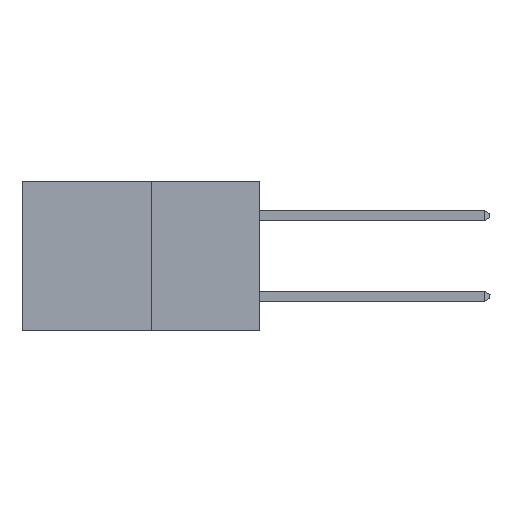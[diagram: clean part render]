
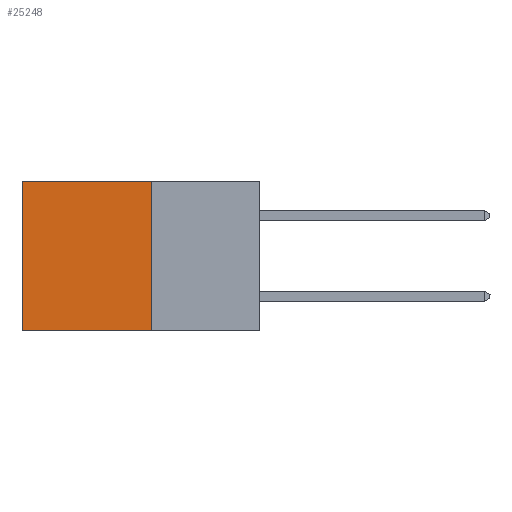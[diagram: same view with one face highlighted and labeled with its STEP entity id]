
A CAD part, left-side view. The second image highlights one B-rep face of the part: STEP entity #25248.
In plain terms, the highlighted planar face has unit normal (-1, 0, 0).
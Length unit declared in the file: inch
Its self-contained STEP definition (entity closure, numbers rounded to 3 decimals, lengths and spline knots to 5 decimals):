
#988 = CARTESIAN_POINT ( 'NONE',  ( 0.277, 0.27, -0.37 ) ) ;
#2246 = VECTOR ( 'NONE', #14841, 39.37008 ) ;
#3165 = AXIS2_PLACEMENT_3D ( 'NONE', #18315, #5723, #20371 ) ;
#3488 = ORIENTED_EDGE ( 'NONE', *, *, #22690, .F. ) ;
#4357 = CARTESIAN_POINT ( 'NONE',  ( 0.277, 0.27, 0. ) ) ;
#5223 = VERTEX_POINT ( 'NONE', #17299 ) ;
#5723 = DIRECTION ( 'NONE',  ( 1., 0., 0. ) ) ;
#6029 = VERTEX_POINT ( 'NONE', #8067 ) ;
#6494 = DIRECTION ( 'NONE',  ( 0., 1., 0. ) ) ;
#6963 = CARTESIAN_POINT ( 'NONE',  ( 0.277, 0.27, -0.37 ) ) ;
#7068 = EDGE_LOOP ( 'NONE', ( #21282, #3488, #13010, #15173 ) ) ;
#7414 = CARTESIAN_POINT ( 'NONE',  ( 0.277, 0.59, -0.37 ) ) ;
#7594 = EDGE_CURVE ( 'NONE', #5223, #8471, #8570, .T. ) ;
#8067 = CARTESIAN_POINT ( 'NONE',  ( 0.277, 0.27, 0. ) ) ;
#8471 = VERTEX_POINT ( 'NONE', #7414 ) ;
#8570 = LINE ( 'NONE', #12725, #2246 ) ;
#9075 = DIRECTION ( 'NONE',  ( 0., 0., -1. ) ) ;
#10999 = VECTOR ( 'NONE', #11600, 39.37008 ) ;
#11600 = DIRECTION ( 'NONE',  ( 0., 1., 0. ) ) ;
#12725 = CARTESIAN_POINT ( 'NONE',  ( 0.277, 0.59, -0.37 ) ) ;
#13010 = ORIENTED_EDGE ( 'NONE', *, *, #18306, .F. ) ;
#13347 = VECTOR ( 'NONE', #6494, 39.37008 ) ;
#14841 = DIRECTION ( 'NONE',  ( 0., 0., -1. ) ) ;
#15173 = ORIENTED_EDGE ( 'NONE', *, *, #24375, .T. ) ;
#17299 = CARTESIAN_POINT ( 'NONE',  ( 0.277, 0.59, 0. ) ) ;
#17780 = VERTEX_POINT ( 'NONE', #24056 ) ;
#18306 = EDGE_CURVE ( 'NONE', #6029, #17780, #21669, .T. ) ;
#18315 = CARTESIAN_POINT ( 'NONE',  ( 0.277, 0.27, -0.37 ) ) ;
#20183 = LINE ( 'NONE', #4357, #13347 ) ;
#20371 = DIRECTION ( 'NONE',  ( 0., 0., -1. ) ) ;
#21015 = VECTOR ( 'NONE', #9075, 39.37008 ) ;
#21282 = ORIENTED_EDGE ( 'NONE', *, *, #7594, .T. ) ;
#21669 = LINE ( 'NONE', #6963, #21015 ) ;
#22690 = EDGE_CURVE ( 'NONE', #17780, #8471, #22694, .T. ) ;
#22694 = LINE ( 'NONE', #988, #10999 ) ;
#23020 = FACE_OUTER_BOUND ( 'NONE', #7068, .T. ) ;
#24056 = CARTESIAN_POINT ( 'NONE',  ( 0.277, 0.27, -0.37 ) ) ;
#24375 = EDGE_CURVE ( 'NONE', #6029, #5223, #20183, .T. ) ;
#24426 = PLANE ( 'NONE',  #3165 ) ;
#25248 = ADVANCED_FACE ( 'NONE', ( #23020 ), #24426, .F. ) ;
